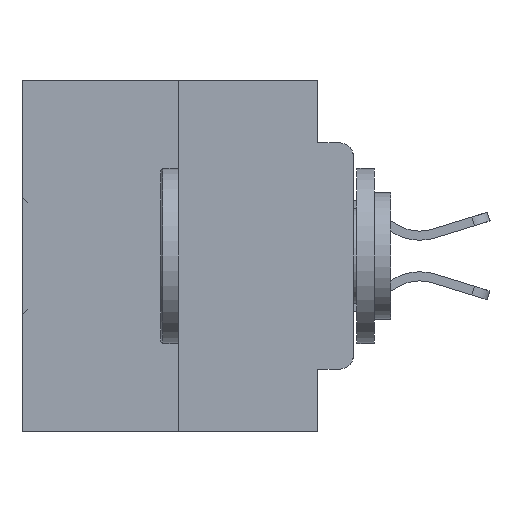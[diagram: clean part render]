
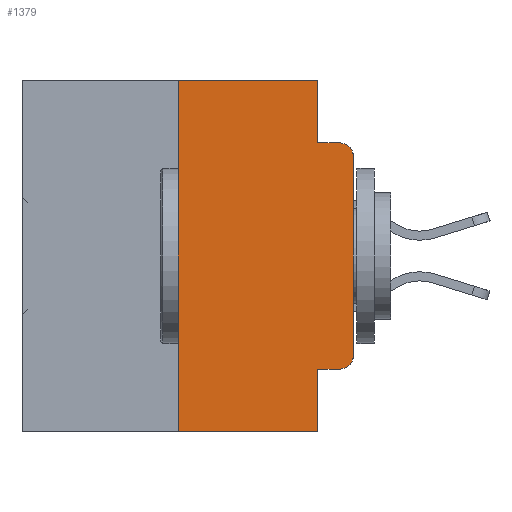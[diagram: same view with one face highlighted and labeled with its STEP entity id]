
A CAD part, left-side view. The second image highlights one B-rep face of the part: STEP entity #1379.
In plain terms, the highlighted planar face has unit normal (-1, 0, 0).
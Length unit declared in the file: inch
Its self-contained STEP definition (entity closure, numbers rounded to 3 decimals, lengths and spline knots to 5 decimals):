
#158 = ORIENTED_EDGE ( 'NONE', *, *, #7596, .T. ) ;
#364 = CARTESIAN_POINT ( 'NONE',  ( 0., 0., 0. ) ) ;
#569 = VERTEX_POINT ( 'NONE', #9394 ) ;
#1081 = DIRECTION ( 'NONE',  ( -1., 0., 0. ) ) ;
#1379 = ADVANCED_FACE ( 'NONE', ( #16646 ), #13595, .F. ) ;
#2359 = EDGE_CURVE ( 'NONE', #21476, #19704, #12039, .T. ) ;
#3132 = VECTOR ( 'NONE', #21736, 39.37008 ) ;
#3486 = VECTOR ( 'NONE', #14226, 39.37008 ) ;
#4687 = EDGE_CURVE ( 'NONE', #10590, #12646, #24779, .T. ) ;
#4765 = LINE ( 'NONE', #15714, #9135 ) ;
#4821 = LINE ( 'NONE', #13439, #23350 ) ;
#4975 = LINE ( 'NONE', #35317, #30091 ) ;
#4990 = DIRECTION ( 'NONE',  ( 0., -1., 0. ) ) ;
#7142 = DIRECTION ( 'NONE',  ( 0., 0., -1. ) ) ;
#7596 = EDGE_CURVE ( 'NONE', #569, #26497, #32309, .T. ) ;
#7664 = LINE ( 'NONE', #18300, #13625 ) ;
#9135 = VECTOR ( 'NONE', #18253, 39.37008 ) ;
#9339 = DIRECTION ( 'NONE',  ( 0., 0., -1. ) ) ;
#9394 = CARTESIAN_POINT ( 'NONE',  ( 0., 0.051, -0.4115 ) ) ;
#10053 = DIRECTION ( 'NONE',  ( 0., -1., 0. ) ) ;
#10430 = CIRCLE ( 'NONE', #30501, 0.02 ) ;
#10590 = VERTEX_POINT ( 'NONE', #27662 ) ;
#10767 = CARTESIAN_POINT ( 'NONE',  ( 0., 0.051, -0.4115 ) ) ;
#11320 = DIRECTION ( 'NONE',  ( 0., 0., 1. ) ) ;
#11345 = AXIS2_PLACEMENT_3D ( 'NONE', #34443, #11838, #7142 ) ;
#11838 = DIRECTION ( 'NONE',  ( -1., 0., 0. ) ) ;
#12039 = LINE ( 'NONE', #33429, #3486 ) ;
#12200 = CARTESIAN_POINT ( 'NONE',  ( 0., 0.02, -0.3915 ) ) ;
#12646 = VERTEX_POINT ( 'NONE', #23547 ) ;
#13303 = VECTOR ( 'NONE', #11320, 39.37008 ) ;
#13439 = CARTESIAN_POINT ( 'NONE',  ( 0., 0.25, 0. ) ) ;
#13595 = PLANE ( 'NONE',  #24245 ) ;
#13625 = VECTOR ( 'NONE', #4990, 39.37008 ) ;
#13971 = ORIENTED_EDGE ( 'NONE', *, *, #34087, .F. ) ;
#14226 = DIRECTION ( 'NONE',  ( 0., -1., 0. ) ) ;
#14550 = EDGE_CURVE ( 'NONE', #26497, #10590, #10430, .T. ) ;
#15714 = CARTESIAN_POINT ( 'NONE',  ( 0., 0.051, 0. ) ) ;
#15900 = VERTEX_POINT ( 'NONE', #17666 ) ;
#16646 = FACE_OUTER_BOUND ( 'NONE', #30090, .T. ) ;
#16808 = CARTESIAN_POINT ( 'NONE',  ( 0., 0.051, -0.0885 ) ) ;
#17666 = CARTESIAN_POINT ( 'NONE',  ( 0., 0.051, -0.5 ) ) ;
#18148 = LINE ( 'NONE', #20677, #35294 ) ;
#18253 = DIRECTION ( 'NONE',  ( 0., 0., -1. ) ) ;
#18285 = VERTEX_POINT ( 'NONE', #35430 ) ;
#18300 = CARTESIAN_POINT ( 'NONE',  ( 0., 0.473, -0.5 ) ) ;
#19174 = DIRECTION ( 'NONE',  ( 0., 0., -1. ) ) ;
#19704 = VERTEX_POINT ( 'NONE', #22358 ) ;
#20542 = CIRCLE ( 'NONE', #11345, 0.02 ) ;
#20677 = CARTESIAN_POINT ( 'NONE',  ( 0., 0.051, -0.0885 ) ) ;
#20865 = ORIENTED_EDGE ( 'NONE', *, *, #4687, .T. ) ;
#21476 = VERTEX_POINT ( 'NONE', #25345 ) ;
#21736 = DIRECTION ( 'NONE',  ( 0., -1., 0. ) ) ;
#21850 = ORIENTED_EDGE ( 'NONE', *, *, #31235, .F. ) ;
#21867 = DIRECTION ( 'NONE',  ( 1., 0., 0. ) ) ;
#22358 = CARTESIAN_POINT ( 'NONE',  ( 0., 0.051, 0. ) ) ;
#22532 = VERTEX_POINT ( 'NONE', #25612 ) ;
#23335 = EDGE_CURVE ( 'NONE', #12646, #22532, #20542, .T. ) ;
#23350 = VECTOR ( 'NONE', #35167, 39.37008 ) ;
#23463 = EDGE_CURVE ( 'NONE', #18285, #15900, #7664, .T. ) ;
#23547 = CARTESIAN_POINT ( 'NONE',  ( 0., 0., -0.1085 ) ) ;
#23697 = ORIENTED_EDGE ( 'NONE', *, *, #31860, .F. ) ;
#23888 = ORIENTED_EDGE ( 'NONE', *, *, #25468, .F. ) ;
#24245 = AXIS2_PLACEMENT_3D ( 'NONE', #26282, #21867, #32800 ) ;
#24779 = LINE ( 'NONE', #364, #13303 ) ;
#25345 = CARTESIAN_POINT ( 'NONE',  ( 0., 0.25, 0. ) ) ;
#25350 = ORIENTED_EDGE ( 'NONE', *, *, #23335, .T. ) ;
#25468 = EDGE_CURVE ( 'NONE', #19704, #34617, #4765, .T. ) ;
#25612 = CARTESIAN_POINT ( 'NONE',  ( 0., 0.02, -0.0885 ) ) ;
#26282 = CARTESIAN_POINT ( 'NONE',  ( 0., 0.473, 0. ) ) ;
#26497 = VERTEX_POINT ( 'NONE', #31984 ) ;
#27662 = CARTESIAN_POINT ( 'NONE',  ( 0., 0., -0.3915 ) ) ;
#27918 = ORIENTED_EDGE ( 'NONE', *, *, #23463, .T. ) ;
#30090 = EDGE_LOOP ( 'NONE', ( #20865, #25350, #21850, #23888, #35176, #13971, #27918, #23697, #158, #30207 ) ) ;
#30091 = VECTOR ( 'NONE', #19174, 39.37008 ) ;
#30207 = ORIENTED_EDGE ( 'NONE', *, *, #14550, .T. ) ;
#30501 = AXIS2_PLACEMENT_3D ( 'NONE', #12200, #1081, #9339 ) ;
#31235 = EDGE_CURVE ( 'NONE', #34617, #22532, #18148, .T. ) ;
#31860 = EDGE_CURVE ( 'NONE', #569, #15900, #4975, .T. ) ;
#31984 = CARTESIAN_POINT ( 'NONE',  ( 0., 0.02, -0.4115 ) ) ;
#32309 = LINE ( 'NONE', #10767, #3132 ) ;
#32800 = DIRECTION ( 'NONE',  ( 0., 0., -1. ) ) ;
#33429 = CARTESIAN_POINT ( 'NONE',  ( 0., 0.473, 0. ) ) ;
#34087 = EDGE_CURVE ( 'NONE', #18285, #21476, #4821, .T. ) ;
#34443 = CARTESIAN_POINT ( 'NONE',  ( 0., 0.02, -0.1085 ) ) ;
#34617 = VERTEX_POINT ( 'NONE', #16808 ) ;
#35167 = DIRECTION ( 'NONE',  ( 0., 0., 1. ) ) ;
#35176 = ORIENTED_EDGE ( 'NONE', *, *, #2359, .F. ) ;
#35294 = VECTOR ( 'NONE', #10053, 39.37008 ) ;
#35317 = CARTESIAN_POINT ( 'NONE',  ( 0., 0.051, 0. ) ) ;
#35430 = CARTESIAN_POINT ( 'NONE',  ( 0., 0.25, -0.5 ) ) ;
